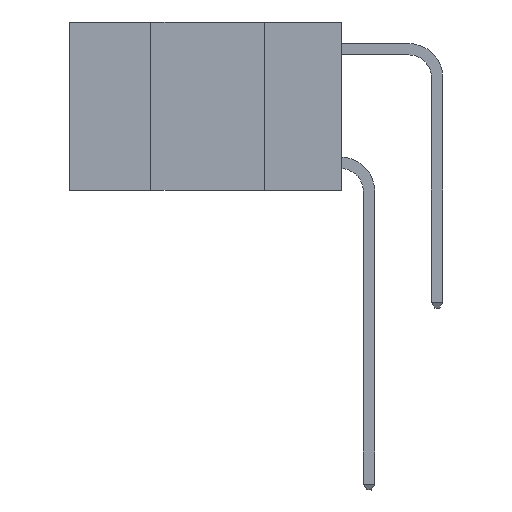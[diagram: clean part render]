
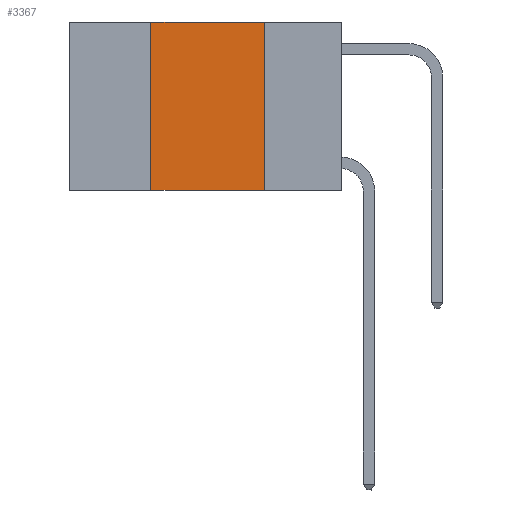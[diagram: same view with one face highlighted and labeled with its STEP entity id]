
A CAD part, left-side view. The second image highlights one B-rep face of the part: STEP entity #3367.
In plain terms, the highlighted planar face has unit normal (-1, 0, 0).
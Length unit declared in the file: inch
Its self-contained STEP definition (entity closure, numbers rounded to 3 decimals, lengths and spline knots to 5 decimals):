
#1323 = CARTESIAN_POINT ( 'NONE',  ( 0., 0.17, 0. ) ) ;
#1386 = LINE ( 'NONE', #20816, #13314 ) ;
#3367 = ADVANCED_FACE ( 'NONE', ( #21177 ), #11492, .F. ) ;
#3719 = EDGE_CURVE ( 'NONE', #20893, #19739, #22571, .T. ) ;
#4898 = EDGE_LOOP ( 'NONE', ( #14454, #6331, #6210, #8440 ) ) ;
#5143 = CARTESIAN_POINT ( 'NONE',  ( 0., 0.42, 0. ) ) ;
#5823 = DIRECTION ( 'NONE',  ( 0., -1., 0. ) ) ;
#6210 = ORIENTED_EDGE ( 'NONE', *, *, #3719, .F. ) ;
#6331 = ORIENTED_EDGE ( 'NONE', *, *, #22137, .F. ) ;
#6592 = VERTEX_POINT ( 'NONE', #7329 ) ;
#7329 = CARTESIAN_POINT ( 'NONE',  ( 0., 0.17, -0.37 ) ) ;
#8440 = ORIENTED_EDGE ( 'NONE', *, *, #10451, .T. ) ;
#8517 = CARTESIAN_POINT ( 'NONE',  ( 0., 0.42, -0.37 ) ) ;
#10451 = EDGE_CURVE ( 'NONE', #20893, #6592, #17410, .T. ) ;
#10834 = VECTOR ( 'NONE', #5823, 39.37008 ) ;
#11140 = LINE ( 'NONE', #16995, #10834 ) ;
#11492 = PLANE ( 'NONE',  #14686 ) ;
#12131 = VECTOR ( 'NONE', #17166, 39.37008 ) ;
#12850 = DIRECTION ( 'NONE',  ( 0., 0., 1. ) ) ;
#13314 = VECTOR ( 'NONE', #14810, 39.37008 ) ;
#13860 = CARTESIAN_POINT ( 'NONE',  ( 0., 0.42, 0. ) ) ;
#14454 = ORIENTED_EDGE ( 'NONE', *, *, #23709, .F. ) ;
#14686 = AXIS2_PLACEMENT_3D ( 'NONE', #19764, #19258, #17357 ) ;
#14810 = DIRECTION ( 'NONE',  ( 0., 0., -1. ) ) ;
#15891 = VERTEX_POINT ( 'NONE', #1323 ) ;
#16775 = VECTOR ( 'NONE', #12850, 39.37008 ) ;
#16995 = CARTESIAN_POINT ( 'NONE',  ( 0., 0.6, 0. ) ) ;
#17166 = DIRECTION ( 'NONE',  ( 0., -1., 0. ) ) ;
#17357 = DIRECTION ( 'NONE',  ( 0., 0., -1. ) ) ;
#17410 = LINE ( 'NONE', #23157, #12131 ) ;
#19258 = DIRECTION ( 'NONE',  ( 1., 0., 0. ) ) ;
#19739 = VERTEX_POINT ( 'NONE', #13860 ) ;
#19764 = CARTESIAN_POINT ( 'NONE',  ( 0., 0.6, 0. ) ) ;
#20816 = CARTESIAN_POINT ( 'NONE',  ( 0., 0.17, 0. ) ) ;
#20893 = VERTEX_POINT ( 'NONE', #8517 ) ;
#21177 = FACE_OUTER_BOUND ( 'NONE', #4898, .T. ) ;
#22137 = EDGE_CURVE ( 'NONE', #19739, #15891, #11140, .T. ) ;
#22571 = LINE ( 'NONE', #5143, #16775 ) ;
#23157 = CARTESIAN_POINT ( 'NONE',  ( 0., 0.6, -0.37 ) ) ;
#23709 = EDGE_CURVE ( 'NONE', #15891, #6592, #1386, .T. ) ;
